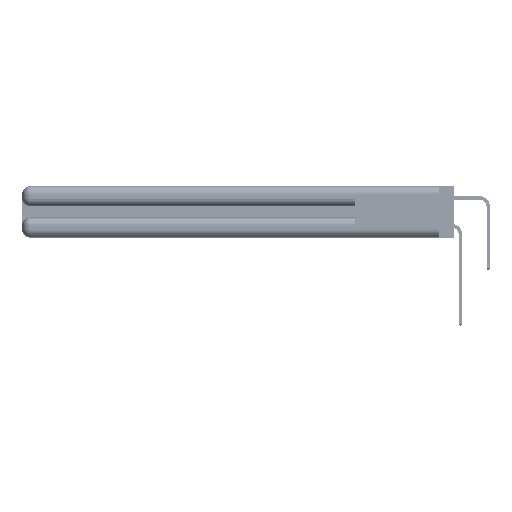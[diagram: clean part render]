
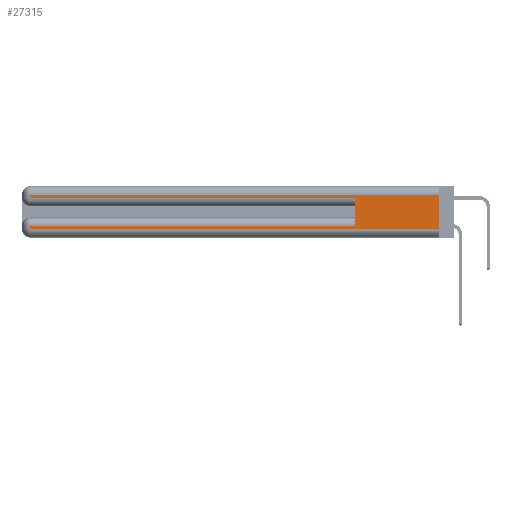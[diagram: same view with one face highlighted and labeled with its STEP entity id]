
A CAD part, left-side view. The second image highlights one B-rep face of the part: STEP entity #27315.
In plain terms, the highlighted planar face has unit normal (-1, 0, 0).
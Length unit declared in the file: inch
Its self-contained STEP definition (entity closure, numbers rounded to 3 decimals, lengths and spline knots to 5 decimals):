
#526 = EDGE_LOOP ( 'NONE', ( #48110, #4591, #17442, #46164, #13572, #31486, #2352, #42294 ) ) ;
#710 = CARTESIAN_POINT ( 'NONE',  ( 0., 0.6, 0.285 ) ) ;
#821 = VECTOR ( 'NONE', #35843, 39.37008 ) ;
#2049 = EDGE_CURVE ( 'NONE', #52449, #40268, #50594, .T. ) ;
#2095 = CARTESIAN_POINT ( 'NONE',  ( 0., 0., 0.31 ) ) ;
#2352 = ORIENTED_EDGE ( 'NONE', *, *, #45192, .T. ) ;
#2391 = VERTEX_POINT ( 'NONE', #20565 ) ;
#2416 = FACE_OUTER_BOUND ( 'NONE', #526, .T. ) ;
#2991 = CARTESIAN_POINT ( 'NONE',  ( 0., 2.94, 0.085 ) ) ;
#3526 = VECTOR ( 'NONE', #42586, 39.37008 ) ;
#4591 = ORIENTED_EDGE ( 'NONE', *, *, #50072, .T. ) ;
#6214 = CARTESIAN_POINT ( 'NONE',  ( 0., 0., 0.085 ) ) ;
#6249 = CARTESIAN_POINT ( 'NONE',  ( 0., 2.94, 0.285 ) ) ;
#6966 = EDGE_CURVE ( 'NONE', #18611, #33330, #33516, .T. ) ;
#11328 = CARTESIAN_POINT ( 'NONE',  ( 0., 2.94, 0.31 ) ) ;
#12625 = VECTOR ( 'NONE', #22208, 39.37008 ) ;
#13024 = CARTESIAN_POINT ( 'NONE',  ( 0., 0., 0.31 ) ) ;
#13572 = ORIENTED_EDGE ( 'NONE', *, *, #36686, .F. ) ;
#15022 = DIRECTION ( 'NONE',  ( 0., 0., -1. ) ) ;
#15486 = CARTESIAN_POINT ( 'NONE',  ( 0., 0., 0.37 ) ) ;
#16178 = VECTOR ( 'NONE', #21295, 39.37008 ) ;
#16326 = VECTOR ( 'NONE', #52575, 39.37008 ) ;
#17442 = ORIENTED_EDGE ( 'NONE', *, *, #50382, .T. ) ;
#17699 = VERTEX_POINT ( 'NONE', #710 ) ;
#18611 = VERTEX_POINT ( 'NONE', #2095 ) ;
#20282 = PLANE ( 'NONE',  #51732 ) ;
#20565 = CARTESIAN_POINT ( 'NONE',  ( 0., 2.94, 0.06 ) ) ;
#21295 = DIRECTION ( 'NONE',  ( 0., 1., 0. ) ) ;
#22208 = DIRECTION ( 'NONE',  ( 0., 0., 1. ) ) ;
#22284 = VERTEX_POINT ( 'NONE', #6249 ) ;
#22349 = LINE ( 'NONE', #39255, #44037 ) ;
#23006 = DIRECTION ( 'NONE',  ( 0., -1., 0. ) ) ;
#23554 = LINE ( 'NONE', #50489, #12625 ) ;
#24371 = DIRECTION ( 'NONE',  ( 1., 0., 0. ) ) ;
#25313 = LINE ( 'NONE', #50564, #3526 ) ;
#27111 = EDGE_CURVE ( 'NONE', #2391, #33330, #22349, .T. ) ;
#27195 = LINE ( 'NONE', #28175, #16326 ) ;
#27315 = ADVANCED_FACE ( 'NONE', ( #2416 ), #20282, .F. ) ;
#28175 = CARTESIAN_POINT ( 'NONE',  ( 0., 2.94, 0.37 ) ) ;
#31486 = ORIENTED_EDGE ( 'NONE', *, *, #2049, .T. ) ;
#33330 = VERTEX_POINT ( 'NONE', #33713 ) ;
#33516 = LINE ( 'NONE', #15486, #821 ) ;
#33713 = CARTESIAN_POINT ( 'NONE',  ( 0., 0., 0.06 ) ) ;
#34688 = LINE ( 'NONE', #39490, #44248 ) ;
#34882 = DIRECTION ( 'NONE',  ( 0., 1., 0. ) ) ;
#35843 = DIRECTION ( 'NONE',  ( 0., 0., -1. ) ) ;
#36686 = EDGE_CURVE ( 'NONE', #52449, #17699, #23554, .T. ) ;
#37770 = EDGE_CURVE ( 'NONE', #22284, #17699, #25313, .T. ) ;
#37885 = LINE ( 'NONE', #13024, #16178 ) ;
#39255 = CARTESIAN_POINT ( 'NONE',  ( 0., 0., 0.06 ) ) ;
#39490 = CARTESIAN_POINT ( 'NONE',  ( 0., 2.94, 0.37 ) ) ;
#40268 = VERTEX_POINT ( 'NONE', #2991 ) ;
#41064 = VECTOR ( 'NONE', #34882, 39.37008 ) ;
#42294 = ORIENTED_EDGE ( 'NONE', *, *, #27111, .T. ) ;
#42586 = DIRECTION ( 'NONE',  ( 0., -1., 0. ) ) ;
#44037 = VECTOR ( 'NONE', #23006, 39.37008 ) ;
#44248 = VECTOR ( 'NONE', #15022, 39.37008 ) ;
#45192 = EDGE_CURVE ( 'NONE', #40268, #2391, #27195, .T. ) ;
#45799 = VERTEX_POINT ( 'NONE', #11328 ) ;
#46164 = ORIENTED_EDGE ( 'NONE', *, *, #37770, .T. ) ;
#48110 = ORIENTED_EDGE ( 'NONE', *, *, #6966, .F. ) ;
#48784 = CARTESIAN_POINT ( 'NONE',  ( 0., 0., 0.37 ) ) ;
#50072 = EDGE_CURVE ( 'NONE', #18611, #45799, #37885, .T. ) ;
#50382 = EDGE_CURVE ( 'NONE', #45799, #22284, #34688, .T. ) ;
#50489 = CARTESIAN_POINT ( 'NONE',  ( 0., 0.6, 0.145 ) ) ;
#50564 = CARTESIAN_POINT ( 'NONE',  ( 0., 0., 0.285 ) ) ;
#50594 = LINE ( 'NONE', #6214, #41064 ) ;
#51732 = AXIS2_PLACEMENT_3D ( 'NONE', #48784, #24371, #52862 ) ;
#52449 = VERTEX_POINT ( 'NONE', #52891 ) ;
#52575 = DIRECTION ( 'NONE',  ( 0., 0., -1. ) ) ;
#52862 = DIRECTION ( 'NONE',  ( 0., 0., -1. ) ) ;
#52891 = CARTESIAN_POINT ( 'NONE',  ( 0., 0.6, 0.085 ) ) ;
